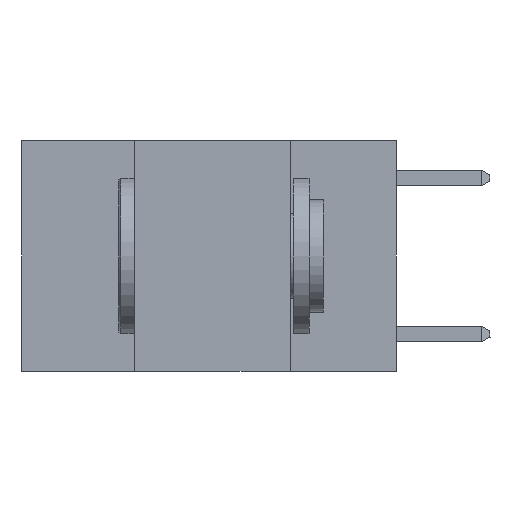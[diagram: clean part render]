
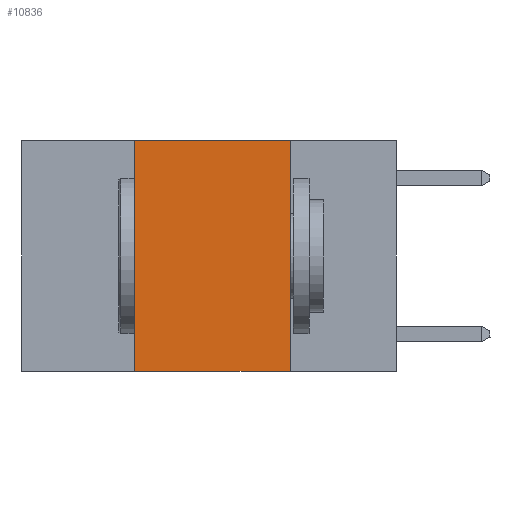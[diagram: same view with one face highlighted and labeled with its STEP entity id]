
A CAD part, left-side view. The second image highlights one B-rep face of the part: STEP entity #10836.
In plain terms, the highlighted planar face has unit normal (-1, 0, 0).
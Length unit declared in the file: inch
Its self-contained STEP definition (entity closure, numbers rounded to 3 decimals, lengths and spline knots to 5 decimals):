
#1173 = VECTOR ( 'NONE', #9778, 39.37008 ) ;
#3021 = CARTESIAN_POINT ( 'NONE',  ( 0., 0.42, 0. ) ) ;
#3343 = LINE ( 'NONE', #5772, #20072 ) ;
#3491 = VERTEX_POINT ( 'NONE', #12837 ) ;
#4662 = VERTEX_POINT ( 'NONE', #13998 ) ;
#5419 = LINE ( 'NONE', #20384, #1173 ) ;
#5597 = DIRECTION ( 'NONE',  ( 1., 0., 0. ) ) ;
#5772 = CARTESIAN_POINT ( 'NONE',  ( 0., 0.6, -0.37 ) ) ;
#6274 = EDGE_CURVE ( 'NONE', #3491, #4662, #15659, .T. ) ;
#8400 = DIRECTION ( 'NONE',  ( 0., 0., -1. ) ) ;
#9443 = CARTESIAN_POINT ( 'NONE',  ( 0., 0.42, 0. ) ) ;
#9778 = DIRECTION ( 'NONE',  ( 0., -1., 0. ) ) ;
#10212 = VERTEX_POINT ( 'NONE', #9443 ) ;
#10836 = ADVANCED_FACE ( 'NONE', ( #20722 ), #16401, .F. ) ;
#12526 = LINE ( 'NONE', #3021, #21293 ) ;
#12837 = CARTESIAN_POINT ( 'NONE',  ( 0., 0.17, 0. ) ) ;
#13998 = CARTESIAN_POINT ( 'NONE',  ( 0., 0.17, -0.37 ) ) ;
#14584 = CARTESIAN_POINT ( 'NONE',  ( 0., 0.6, 0. ) ) ;
#15201 = AXIS2_PLACEMENT_3D ( 'NONE', #14584, #5597, #18133 ) ;
#15635 = VECTOR ( 'NONE', #8400, 39.37008 ) ;
#15659 = LINE ( 'NONE', #22362, #15635 ) ;
#16401 = PLANE ( 'NONE',  #15201 ) ;
#17109 = VERTEX_POINT ( 'NONE', #19818 ) ;
#17544 = EDGE_CURVE ( 'NONE', #17109, #10212, #12526, .T. ) ;
#18133 = DIRECTION ( 'NONE',  ( 0., 0., -1. ) ) ;
#18904 = EDGE_LOOP ( 'NONE', ( #20468, #20506, #20613, #20666 ) ) ;
#19037 = DIRECTION ( 'NONE',  ( 0., 0., 1. ) ) ;
#19062 = EDGE_CURVE ( 'NONE', #10212, #3491, #5419, .T. ) ;
#19818 = CARTESIAN_POINT ( 'NONE',  ( 0., 0.42, -0.37 ) ) ;
#20072 = VECTOR ( 'NONE', #21763, 39.37008 ) ;
#20384 = CARTESIAN_POINT ( 'NONE',  ( 0., 0.6, 0. ) ) ;
#20468 = ORIENTED_EDGE ( 'NONE', *, *, #6274, .F. ) ;
#20506 = ORIENTED_EDGE ( 'NONE', *, *, #19062, .F. ) ;
#20613 = ORIENTED_EDGE ( 'NONE', *, *, #17544, .F. ) ;
#20666 = ORIENTED_EDGE ( 'NONE', *, *, #22057, .T. ) ;
#20722 = FACE_OUTER_BOUND ( 'NONE', #18904, .T. ) ;
#21293 = VECTOR ( 'NONE', #19037, 39.37008 ) ;
#21763 = DIRECTION ( 'NONE',  ( 0., -1., 0. ) ) ;
#22057 = EDGE_CURVE ( 'NONE', #17109, #4662, #3343, .T. ) ;
#22362 = CARTESIAN_POINT ( 'NONE',  ( 0., 0.17, 0. ) ) ;
